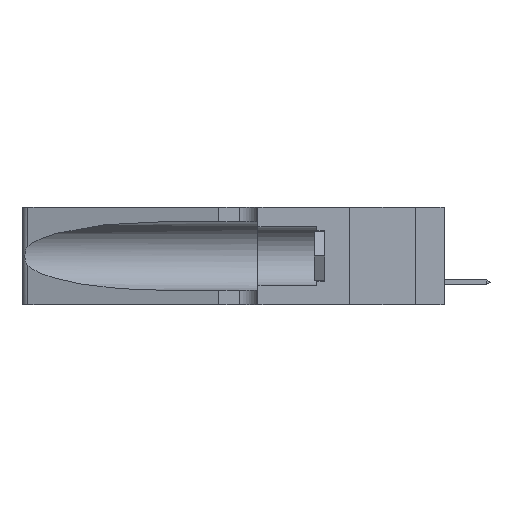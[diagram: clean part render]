
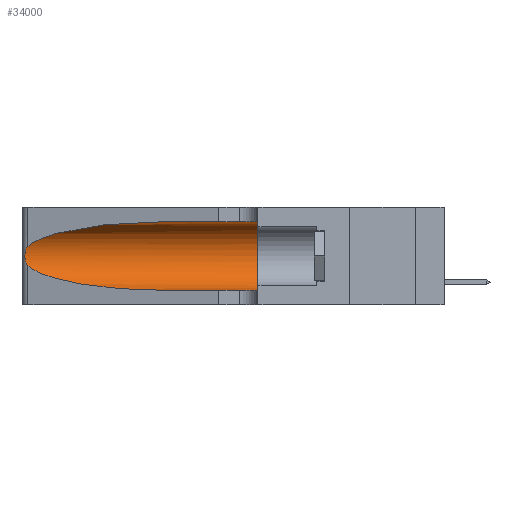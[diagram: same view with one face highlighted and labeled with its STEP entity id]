
A CAD part, left-side view. The second image highlights one B-rep face of the part: STEP entity #34000.
In plain terms, the highlighted cylindrical face has radius 3.308 mm (diameter 6.617 mm), a partial arc.
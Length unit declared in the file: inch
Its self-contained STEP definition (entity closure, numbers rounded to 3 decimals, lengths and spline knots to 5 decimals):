
#49 = CARTESIAN_POINT ( 'NONE',  ( 0.26018, 1.23835, 0.19895 ) ) ;
#1014 = ORIENTED_EDGE ( 'NONE', *, *, #44471, .T. ) ;
#2190 = CARTESIAN_POINT ( 'NONE',  ( 0.2373, 1.15595, 0.28018 ) ) ;
#3456 = CARTESIAN_POINT ( 'NONE',  ( 0.25487, 1.22718, 0.22369 ) ) ;
#3521 = VECTOR ( 'NONE', #13329, 39.37008 ) ;
#3604 = CARTESIAN_POINT ( 'NONE',  ( 0.25555, 1.22993, 0.14849 ) ) ;
#4262 = VERTEX_POINT ( 'NONE', #40715 ) ;
#5119 = ORIENTED_EDGE ( 'NONE', *, *, #25184, .F. ) ;
#5354 = CYLINDRICAL_SURFACE ( 'NONE', #28834, 0.13025 ) ;
#5507 = CARTESIAN_POINT ( 'NONE',  ( 0.25487, 1.22718, 0.22369 ) ) ;
#6023 = CARTESIAN_POINT ( 'NONE',  ( 0.2373, 1.15595, 0.08982 ) ) ;
#7231 = CARTESIAN_POINT ( 'NONE',  ( 0.25787, 1.23484, 0.2124 ) ) ;
#8436 = EDGE_CURVE ( 'NONE', #19063, #10226, #23371, .T. ) ;
#8499 = VERTEX_POINT ( 'NONE', #20501 ) ;
#9325 = CARTESIAN_POINT ( 'NONE',  ( 0.25487, 1.22718, 0.14631 ) ) ;
#9701 = AXIS2_PLACEMENT_3D ( 'NONE', #22817, #37885, #23133 ) ;
#10226 = VERTEX_POINT ( 'NONE', #34184 ) ;
#10268 = EDGE_LOOP ( 'NONE', ( #40391, #23958, #1014, #27035, #5119, #13331 ) ) ;
#10549 = CARTESIAN_POINT ( 'NONE',  ( 0.25639, 1.23184, 0.21858 ) ) ;
#10699 = CARTESIAN_POINT ( 'NONE',  ( 0.25789, 1.23486, 0.15765 ) ) ;
#10985 = CARTESIAN_POINT ( 'NONE',  ( 0.26017, 1.23833, 0.17102 ) ) ;
#11716 = VERTEX_POINT ( 'NONE', #38512 ) ;
#13308 = VECTOR ( 'NONE', #32413, 39.37008 ) ;
#13329 = DIRECTION ( 'NONE',  ( 0., -1., 0. ) ) ;
#13331 = ORIENTED_EDGE ( 'NONE', *, *, #31052, .F. ) ;
#13846 = CARTESIAN_POINT ( 'NONE',  ( 0.1305, 1.61858, 0.185 ) ) ;
#14085 = CARTESIAN_POINT ( 'NONE',  ( 0.1305, 0.72297, 0.05475 ) ) ;
#16486 = DIRECTION ( 'NONE',  ( 0., 0., -1. ) ) ;
#18714 = FACE_OUTER_BOUND ( 'NONE', #10268, .T. ) ;
#19063 = VERTEX_POINT ( 'NONE', #14085 ) ;
#20370 = CARTESIAN_POINT ( 'NONE',  ( 0.18966, 0.96281, 0.31525 ) ) ;
#20501 = CARTESIAN_POINT ( 'NONE',  ( 0.1305, 0.72297, 0.31525 ) ) ;
#22817 = CARTESIAN_POINT ( 'NONE',  ( 0.1305, 0.35, 0.185 ) ) ;
#23133 = DIRECTION ( 'NONE',  ( 0., 0., 1. ) ) ;
#23371 = LINE ( 'NONE', #42288, #13308 ) ;
#23958 = ORIENTED_EDGE ( 'NONE', *, *, #39093, .T. ) ;
#24962 = CARTESIAN_POINT ( 'NONE',  ( 0.26075, 1.23896, 0.178 ) ) ;
#25105 = CARTESIAN_POINT ( 'NONE',  ( 0.26075, 1.23896, 0.19203 ) ) ;
#25184 = EDGE_CURVE ( 'NONE', #11716, #10226, #29642, .T. ) ;
#26117 =( BOUNDED_CURVE ( )  B_SPLINE_CURVE ( 3, ( #9325, #6023, #34404, #41908 ),
 .UNSPECIFIED., .F., .T. ) 
 B_SPLINE_CURVE_WITH_KNOTS ( ( 4, 4 ),
 ( 3.44316, 4.71239 ),
 .UNSPECIFIED. ) 
 CURVE ( )  GEOMETRIC_REPRESENTATION_ITEM ( )  RATIONAL_B_SPLINE_CURVE ( ( 1., 0.87, 0.87, 1. ) ) 
 REPRESENTATION_ITEM ( '' )  );
#27035 = ORIENTED_EDGE ( 'NONE', *, *, #8436, .T. ) ;
#27461 = DIRECTION ( 'NONE',  ( 0., -1., 0. ) ) ;
#27606 = CARTESIAN_POINT ( 'NONE',  ( 0.1305, 1.61858, 0.31525 ) ) ;
#28411 = CARTESIAN_POINT ( 'NONE',  ( 0.25555, 1.22994, 0.2215 ) ) ;
#28834 = AXIS2_PLACEMENT_3D ( 'NONE', #13846, #27461, #16486 ) ;
#29642 = CIRCLE ( 'NONE', #9701, 0.13025 ) ;
#30164 =( BOUNDED_CURVE ( )  B_SPLINE_CURVE ( 3, ( #30587, #20370, #2190, #5507 ),
 .UNSPECIFIED., .F., .T. ) 
 B_SPLINE_CURVE_WITH_KNOTS ( ( 4, 4 ),
 ( 1.5708, 2.84003 ),
 .UNSPECIFIED. ) 
 CURVE ( )  GEOMETRIC_REPRESENTATION_ITEM ( )  RATIONAL_B_SPLINE_CURVE ( ( 1., 0.87, 0.87, 1. ) ) 
 REPRESENTATION_ITEM ( '' )  );
#30587 = CARTESIAN_POINT ( 'NONE',  ( 0.1305, 0.72297, 0.31525 ) ) ;
#30845 = EDGE_CURVE ( 'NONE', #8499, #32035, #30164, .T. ) ;
#31052 = EDGE_CURVE ( 'NONE', #8499, #11716, #43884, .T. ) ;
#32026 = CARTESIAN_POINT ( 'NONE',  ( 0.25487, 1.22718, 0.22369 ) ) ;
#32035 = VERTEX_POINT ( 'NONE', #32026 ) ;
#32178 = CARTESIAN_POINT ( 'NONE',  ( 0.25856, 1.23593, 0.16098 ) ) ;
#32413 = DIRECTION ( 'NONE',  ( 0., -1., 0. ) ) ;
#34000 = ADVANCED_FACE ( 'NONE', ( #18714 ), #5354, .F. ) ;
#34184 = CARTESIAN_POINT ( 'NONE',  ( 0.1305, 0.35, 0.05475 ) ) ;
#34404 = CARTESIAN_POINT ( 'NONE',  ( 0.18966, 0.96281, 0.05475 ) ) ;
#34521 = B_SPLINE_CURVE_WITH_KNOTS ( 'NONE', 3,
 ( #3456, #28411, #10549, #7231, #35647, #49, #25105, #24962, #10985, #32178, #10699, #35783, #3604, #36047 ),
 .UNSPECIFIED., .F., .F.,
 ( 4, 2, 2, 2, 2, 2, 4 ),
 ( 0., 0.00027, 0.00053, 0.00107, 0.0016, 0.00187, 0.00214 ),
 .UNSPECIFIED. ) ;
#35647 = CARTESIAN_POINT ( 'NONE',  ( 0.25854, 1.2359, 0.20912 ) ) ;
#35783 = CARTESIAN_POINT ( 'NONE',  ( 0.25639, 1.23186, 0.15144 ) ) ;
#36047 = CARTESIAN_POINT ( 'NONE',  ( 0.25487, 1.22718, 0.14631 ) ) ;
#37885 = DIRECTION ( 'NONE',  ( 0., 1., 0. ) ) ;
#38512 = CARTESIAN_POINT ( 'NONE',  ( 0.1305, 0.35, 0.31525 ) ) ;
#39093 = EDGE_CURVE ( 'NONE', #32035, #4262, #34521, .T. ) ;
#40391 = ORIENTED_EDGE ( 'NONE', *, *, #30845, .T. ) ;
#40715 = CARTESIAN_POINT ( 'NONE',  ( 0.25487, 1.22718, 0.14631 ) ) ;
#41908 = CARTESIAN_POINT ( 'NONE',  ( 0.1305, 0.72297, 0.05475 ) ) ;
#42288 = CARTESIAN_POINT ( 'NONE',  ( 0.1305, 1.61858, 0.05475 ) ) ;
#43884 = LINE ( 'NONE', #27606, #3521 ) ;
#44471 = EDGE_CURVE ( 'NONE', #4262, #19063, #26117, .T. ) ;
